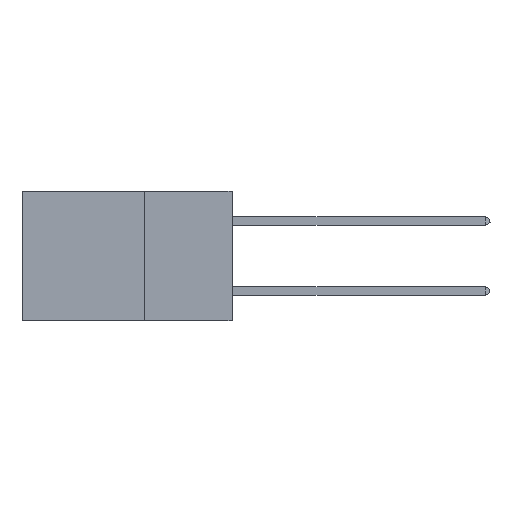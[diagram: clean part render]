
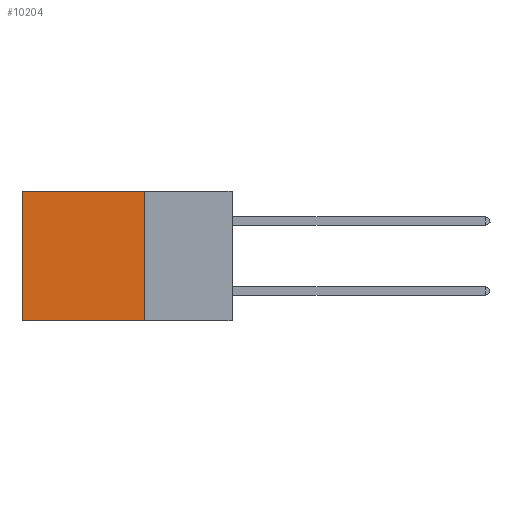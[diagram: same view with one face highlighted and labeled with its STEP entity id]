
A CAD part, left-side view. The second image highlights one B-rep face of the part: STEP entity #10204.
In plain terms, the highlighted planar face has unit normal (-1, 0, 0).
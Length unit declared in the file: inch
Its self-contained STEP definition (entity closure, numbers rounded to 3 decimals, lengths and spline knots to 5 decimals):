
#809 = CARTESIAN_POINT ( 'NONE',  ( 0.2875, 0.25, 0. ) ) ;
#1191 = DIRECTION ( 'NONE',  ( 0., 0., -1. ) ) ;
#1272 = VECTOR ( 'NONE', #12809, 39.37008 ) ;
#1781 = CARTESIAN_POINT ( 'NONE',  ( 0.2875, 0.25, 0. ) ) ;
#3431 = PLANE ( 'NONE',  #9731 ) ;
#3482 = CARTESIAN_POINT ( 'NONE',  ( 0.2875, 0.25, 0. ) ) ;
#3741 = EDGE_CURVE ( 'NONE', #12913, #19523, #18429, .T. ) ;
#5404 = VERTEX_POINT ( 'NONE', #13031 ) ;
#6002 = EDGE_CURVE ( 'NONE', #5404, #12929, #9597, .T. ) ;
#6366 = LINE ( 'NONE', #17884, #10451 ) ;
#6852 = DIRECTION ( 'NONE',  ( 0., 0., -1. ) ) ;
#7869 = LINE ( 'NONE', #13026, #1272 ) ;
#7954 = CARTESIAN_POINT ( 'NONE',  ( 0.2875, 0.25, -0.37 ) ) ;
#8117 = DIRECTION ( 'NONE',  ( 0., 1., 0. ) ) ;
#8494 = DIRECTION ( 'NONE',  ( 1., 0., 0. ) ) ;
#9597 = LINE ( 'NONE', #7954, #12572 ) ;
#9731 = AXIS2_PLACEMENT_3D ( 'NONE', #1781, #8494, #6852 ) ;
#9794 = EDGE_LOOP ( 'NONE', ( #18552, #14114, #21538, #12248 ) ) ;
#10204 = ADVANCED_FACE ( 'NONE', ( #12324 ), #3431, .F. ) ;
#10451 = VECTOR ( 'NONE', #1191, 39.37008 ) ;
#11278 = EDGE_CURVE ( 'NONE', #19523, #12929, #7869, .T. ) ;
#12181 = EDGE_CURVE ( 'NONE', #12913, #5404, #6366, .T. ) ;
#12248 = ORIENTED_EDGE ( 'NONE', *, *, #3741, .T. ) ;
#12324 = FACE_OUTER_BOUND ( 'NONE', #9794, .T. ) ;
#12572 = VECTOR ( 'NONE', #14637, 39.37008 ) ;
#12809 = DIRECTION ( 'NONE',  ( 0., 0., -1. ) ) ;
#12913 = VERTEX_POINT ( 'NONE', #809 ) ;
#12929 = VERTEX_POINT ( 'NONE', #17190 ) ;
#13026 = CARTESIAN_POINT ( 'NONE',  ( 0.2875, 0.6, 0. ) ) ;
#13031 = CARTESIAN_POINT ( 'NONE',  ( 0.2875, 0.25, -0.37 ) ) ;
#14114 = ORIENTED_EDGE ( 'NONE', *, *, #6002, .F. ) ;
#14637 = DIRECTION ( 'NONE',  ( 0., 1., 0. ) ) ;
#14973 = CARTESIAN_POINT ( 'NONE',  ( 0.2875, 0.6, 0. ) ) ;
#17190 = CARTESIAN_POINT ( 'NONE',  ( 0.2875, 0.6, -0.37 ) ) ;
#17884 = CARTESIAN_POINT ( 'NONE',  ( 0.2875, 0.25, 0. ) ) ;
#18429 = LINE ( 'NONE', #3482, #20138 ) ;
#18552 = ORIENTED_EDGE ( 'NONE', *, *, #11278, .T. ) ;
#19523 = VERTEX_POINT ( 'NONE', #14973 ) ;
#20138 = VECTOR ( 'NONE', #8117, 39.37008 ) ;
#21538 = ORIENTED_EDGE ( 'NONE', *, *, #12181, .F. ) ;
